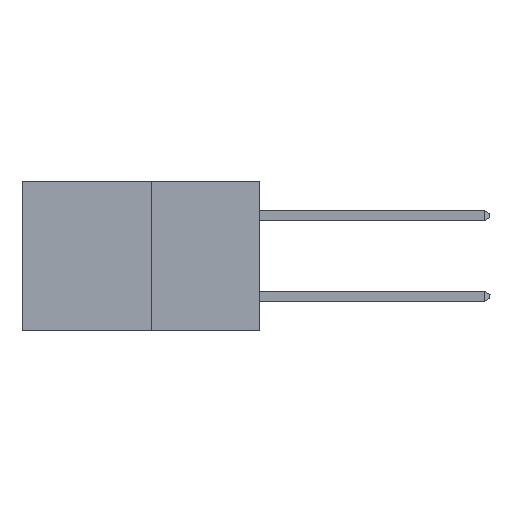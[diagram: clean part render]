
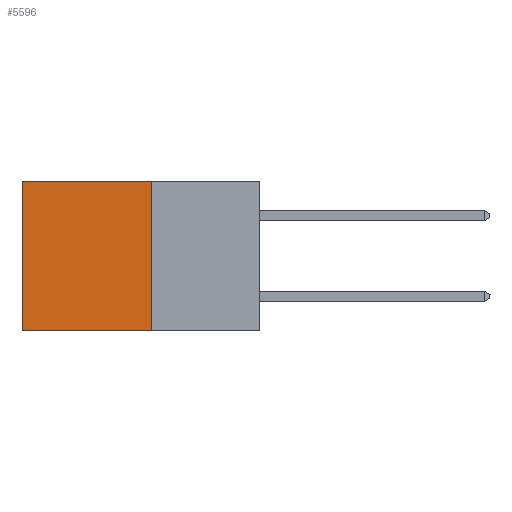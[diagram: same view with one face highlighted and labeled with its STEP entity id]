
A CAD part, left-side view. The second image highlights one B-rep face of the part: STEP entity #5596.
In plain terms, the highlighted planar face has unit normal (-1, 0, 0).
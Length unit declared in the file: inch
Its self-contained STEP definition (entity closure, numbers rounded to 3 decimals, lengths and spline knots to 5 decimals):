
#806 = DIRECTION ( 'NONE',  ( 0., 0., -1. ) ) ;
#835 = CARTESIAN_POINT ( 'NONE',  ( 0.277, 0.27, -0.37 ) ) ;
#1286 = VECTOR ( 'NONE', #806, 39.37008 ) ;
#1313 = EDGE_CURVE ( 'NONE', #1329, #5897, #5960, .T. ) ;
#1329 = VERTEX_POINT ( 'NONE', #7607 ) ;
#1473 = ORIENTED_EDGE ( 'NONE', *, *, #6432, .F. ) ;
#1658 = EDGE_CURVE ( 'NONE', #5897, #8981, #7393, .T. ) ;
#2210 = VECTOR ( 'NONE', #8728, 39.37008 ) ;
#3642 = DIRECTION ( 'NONE',  ( 0., 1., 0. ) ) ;
#3844 = ORIENTED_EDGE ( 'NONE', *, *, #1313, .T. ) ;
#3855 = ORIENTED_EDGE ( 'NONE', *, *, #1658, .T. ) ;
#3915 = CARTESIAN_POINT ( 'NONE',  ( 0.277, 0.59, 0. ) ) ;
#4942 = VERTEX_POINT ( 'NONE', #10375 ) ;
#5173 = EDGE_CURVE ( 'NONE', #4942, #8981, #11611, .T. ) ;
#5596 = ADVANCED_FACE ( 'NONE', ( #9025 ), #5680, .F. ) ;
#5638 = DIRECTION ( 'NONE',  ( 0., 0., -1. ) ) ;
#5648 = DIRECTION ( 'NONE',  ( 1., 0., 0. ) ) ;
#5680 = PLANE ( 'NONE',  #11787 ) ;
#5796 = CARTESIAN_POINT ( 'NONE',  ( 0.277, 0.27, -0.37 ) ) ;
#5897 = VERTEX_POINT ( 'NONE', #3915 ) ;
#5960 = LINE ( 'NONE', #6659, #10374 ) ;
#6432 = EDGE_CURVE ( 'NONE', #1329, #4942, #10898, .T. ) ;
#6434 = ORIENTED_EDGE ( 'NONE', *, *, #5173, .F. ) ;
#6659 = CARTESIAN_POINT ( 'NONE',  ( 0.277, 0.27, 0. ) ) ;
#7393 = LINE ( 'NONE', #10232, #2210 ) ;
#7607 = CARTESIAN_POINT ( 'NONE',  ( 0.277, 0.27, 0. ) ) ;
#8728 = DIRECTION ( 'NONE',  ( 0., 0., -1. ) ) ;
#8923 = EDGE_LOOP ( 'NONE', ( #3855, #6434, #1473, #3844 ) ) ;
#8937 = CARTESIAN_POINT ( 'NONE',  ( 0.277, 0.27, -0.37 ) ) ;
#8952 = DIRECTION ( 'NONE',  ( 0., 1., 0. ) ) ;
#8981 = VERTEX_POINT ( 'NONE', #10075 ) ;
#9025 = FACE_OUTER_BOUND ( 'NONE', #8923, .T. ) ;
#9035 = VECTOR ( 'NONE', #8952, 39.37008 ) ;
#10075 = CARTESIAN_POINT ( 'NONE',  ( 0.277, 0.59, -0.37 ) ) ;
#10232 = CARTESIAN_POINT ( 'NONE',  ( 0.277, 0.59, -0.37 ) ) ;
#10374 = VECTOR ( 'NONE', #3642, 39.37008 ) ;
#10375 = CARTESIAN_POINT ( 'NONE',  ( 0.277, 0.27, -0.37 ) ) ;
#10898 = LINE ( 'NONE', #835, #1286 ) ;
#11611 = LINE ( 'NONE', #8937, #9035 ) ;
#11787 = AXIS2_PLACEMENT_3D ( 'NONE', #5796, #5648, #5638 ) ;
